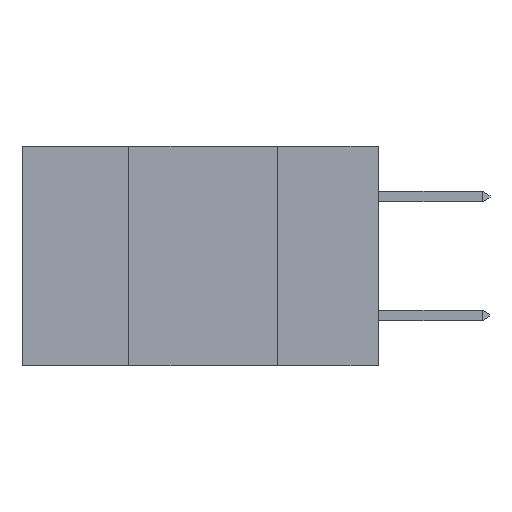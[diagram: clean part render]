
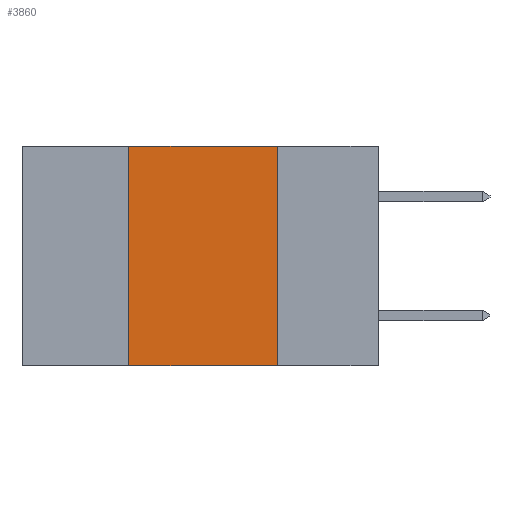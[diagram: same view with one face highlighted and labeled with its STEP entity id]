
A CAD part, left-side view. The second image highlights one B-rep face of the part: STEP entity #3860.
In plain terms, the highlighted planar face has unit normal (-1, 0, 0).
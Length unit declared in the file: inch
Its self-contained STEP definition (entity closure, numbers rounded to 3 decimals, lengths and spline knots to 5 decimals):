
#242 = CARTESIAN_POINT ( 'NONE',  ( 0., 0.42, 0. ) ) ;
#322 = CARTESIAN_POINT ( 'NONE',  ( 0., 0.6, 0. ) ) ;
#418 = FACE_OUTER_BOUND ( 'NONE', #2296, .T. ) ;
#546 = CARTESIAN_POINT ( 'NONE',  ( 0., 0.17, 0. ) ) ;
#559 = VERTEX_POINT ( 'NONE', #6033 ) ;
#581 = VERTEX_POINT ( 'NONE', #2435 ) ;
#1225 = DIRECTION ( 'NONE',  ( 0., -1., 0. ) ) ;
#1342 = CARTESIAN_POINT ( 'NONE',  ( 0., 0.6, -0.37 ) ) ;
#1848 = CARTESIAN_POINT ( 'NONE',  ( 0., 0.17, 0. ) ) ;
#2296 = EDGE_LOOP ( 'NONE', ( #9363, #10697, #11147, #5250 ) ) ;
#2378 = VECTOR ( 'NONE', #4645, 39.37008 ) ;
#2435 = CARTESIAN_POINT ( 'NONE',  ( 0., 0.42, 0. ) ) ;
#3776 = DIRECTION ( 'NONE',  ( 1., 0., 0. ) ) ;
#3805 = PLANE ( 'NONE',  #11035 ) ;
#3860 = ADVANCED_FACE ( 'NONE', ( #418 ), #3805, .F. ) ;
#4090 = LINE ( 'NONE', #242, #6805 ) ;
#4502 = VECTOR ( 'NONE', #1225, 39.37008 ) ;
#4645 = DIRECTION ( 'NONE',  ( 0., 0., -1. ) ) ;
#4850 = LINE ( 'NONE', #322, #9193 ) ;
#4920 = EDGE_CURVE ( 'NONE', #559, #581, #4090, .T. ) ;
#5054 = EDGE_CURVE ( 'NONE', #581, #5426, #4850, .T. ) ;
#5059 = LINE ( 'NONE', #1342, #4502 ) ;
#5250 = ORIENTED_EDGE ( 'NONE', *, *, #7079, .T. ) ;
#5426 = VERTEX_POINT ( 'NONE', #546 ) ;
#6033 = CARTESIAN_POINT ( 'NONE',  ( 0., 0.42, -0.37 ) ) ;
#6295 = CARTESIAN_POINT ( 'NONE',  ( 0., 0.6, 0. ) ) ;
#6805 = VECTOR ( 'NONE', #6895, 39.37008 ) ;
#6895 = DIRECTION ( 'NONE',  ( 0., 0., 1. ) ) ;
#7079 = EDGE_CURVE ( 'NONE', #559, #9225, #5059, .T. ) ;
#8226 = DIRECTION ( 'NONE',  ( 0., -1., 0. ) ) ;
#9141 = EDGE_CURVE ( 'NONE', #5426, #9225, #9494, .T. ) ;
#9193 = VECTOR ( 'NONE', #8226, 39.37008 ) ;
#9225 = VERTEX_POINT ( 'NONE', #10789 ) ;
#9363 = ORIENTED_EDGE ( 'NONE', *, *, #9141, .F. ) ;
#9494 = LINE ( 'NONE', #1848, #2378 ) ;
#10697 = ORIENTED_EDGE ( 'NONE', *, *, #5054, .F. ) ;
#10789 = CARTESIAN_POINT ( 'NONE',  ( 0., 0.17, -0.37 ) ) ;
#11035 = AXIS2_PLACEMENT_3D ( 'NONE', #6295, #3776, #11299 ) ;
#11147 = ORIENTED_EDGE ( 'NONE', *, *, #4920, .F. ) ;
#11299 = DIRECTION ( 'NONE',  ( 0., 0., -1. ) ) ;
